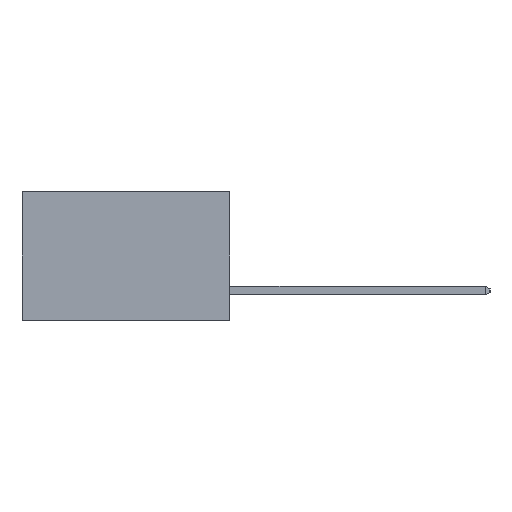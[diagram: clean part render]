
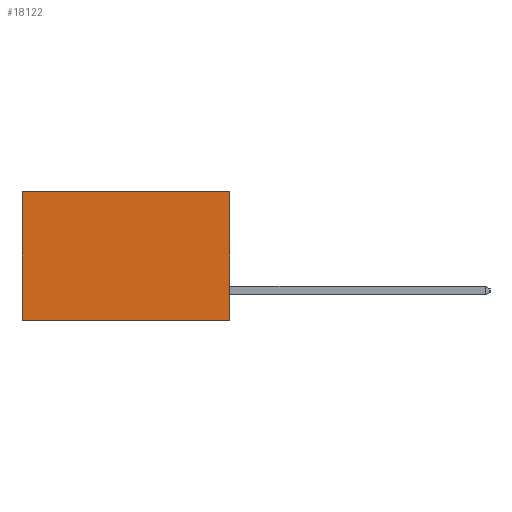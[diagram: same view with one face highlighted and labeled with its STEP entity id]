
A CAD part, left-side view. The second image highlights one B-rep face of the part: STEP entity #18122.
In plain terms, the highlighted planar face has unit normal (-1, 0, 0).
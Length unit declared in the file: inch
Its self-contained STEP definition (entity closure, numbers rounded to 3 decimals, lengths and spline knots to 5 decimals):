
#447 = LINE ( 'NONE', #11173, #11490 ) ;
#457 = CARTESIAN_POINT ( 'NONE',  ( 0.298, 0., 0. ) ) ;
#874 = VECTOR ( 'NONE', #12557, 39.37008 ) ;
#1066 = VECTOR ( 'NONE', #4294, 39.37008 ) ;
#1334 = LINE ( 'NONE', #18081, #874 ) ;
#1494 = CARTESIAN_POINT ( 'NONE',  ( 0.298, 0.6, -0.37 ) ) ;
#1973 = DIRECTION ( 'NONE',  ( 0., 0., -1. ) ) ;
#2260 = VECTOR ( 'NONE', #6563, 39.37008 ) ;
#2614 = DIRECTION ( 'NONE',  ( 0., 0., -1. ) ) ;
#2716 = LINE ( 'NONE', #13586, #2260 ) ;
#2901 = ORIENTED_EDGE ( 'NONE', *, *, #17050, .F. ) ;
#4294 = DIRECTION ( 'NONE',  ( 0., 1., 0. ) ) ;
#4640 = VERTEX_POINT ( 'NONE', #13019 ) ;
#6563 = DIRECTION ( 'NONE',  ( 0., 1., 0. ) ) ;
#7437 = FACE_OUTER_BOUND ( 'NONE', #11587, .T. ) ;
#7696 = PLANE ( 'NONE',  #13931 ) ;
#8779 = LINE ( 'NONE', #11399, #1066 ) ;
#9036 = EDGE_CURVE ( 'NONE', #4640, #16682, #447, .T. ) ;
#10559 = DIRECTION ( 'NONE',  ( 1., 0., 0. ) ) ;
#11173 = CARTESIAN_POINT ( 'NONE',  ( 0.298, 0.6, 0. ) ) ;
#11399 = CARTESIAN_POINT ( 'NONE',  ( 0.298, 0., -0.37 ) ) ;
#11490 = VECTOR ( 'NONE', #2614, 39.37008 ) ;
#11587 = EDGE_LOOP ( 'NONE', ( #17572, #13568, #2901, #12732 ) ) ;
#12557 = DIRECTION ( 'NONE',  ( 0., 0., -1. ) ) ;
#12656 = CARTESIAN_POINT ( 'NONE',  ( 0.298, 0., 0. ) ) ;
#12732 = ORIENTED_EDGE ( 'NONE', *, *, #16968, .T. ) ;
#13019 = CARTESIAN_POINT ( 'NONE',  ( 0.298, 0.6, 0. ) ) ;
#13069 = CARTESIAN_POINT ( 'NONE',  ( 0.298, 0., -0.37 ) ) ;
#13479 = VERTEX_POINT ( 'NONE', #13069 ) ;
#13568 = ORIENTED_EDGE ( 'NONE', *, *, #18452, .F. ) ;
#13586 = CARTESIAN_POINT ( 'NONE',  ( 0.298, 0., 0. ) ) ;
#13931 = AXIS2_PLACEMENT_3D ( 'NONE', #457, #10559, #1973 ) ;
#16682 = VERTEX_POINT ( 'NONE', #1494 ) ;
#16968 = EDGE_CURVE ( 'NONE', #17801, #4640, #2716, .T. ) ;
#17050 = EDGE_CURVE ( 'NONE', #17801, #13479, #1334, .T. ) ;
#17572 = ORIENTED_EDGE ( 'NONE', *, *, #9036, .T. ) ;
#17801 = VERTEX_POINT ( 'NONE', #12656 ) ;
#18081 = CARTESIAN_POINT ( 'NONE',  ( 0.298, 0., 0. ) ) ;
#18122 = ADVANCED_FACE ( 'NONE', ( #7437 ), #7696, .F. ) ;
#18452 = EDGE_CURVE ( 'NONE', #13479, #16682, #8779, .T. ) ;
